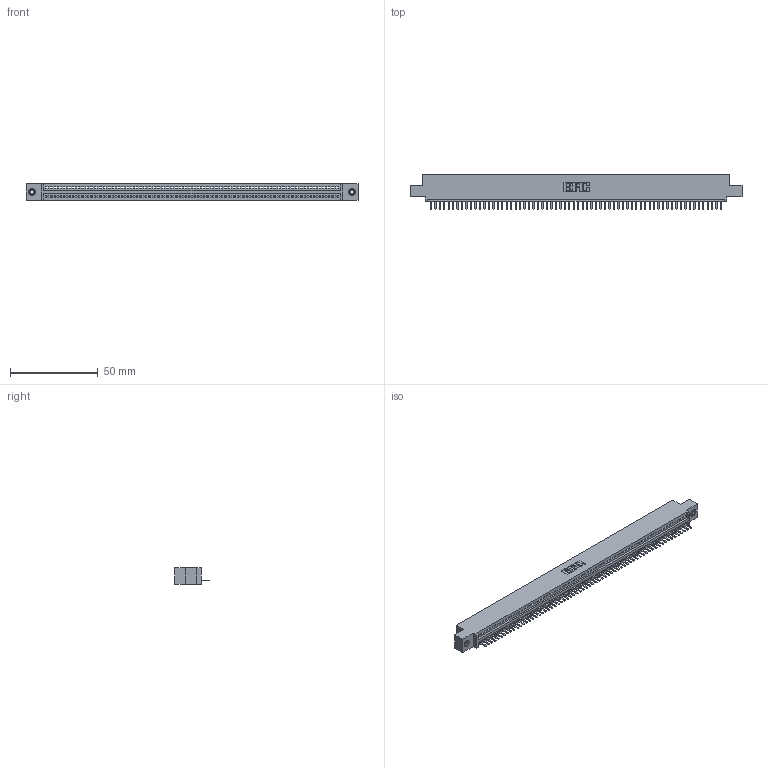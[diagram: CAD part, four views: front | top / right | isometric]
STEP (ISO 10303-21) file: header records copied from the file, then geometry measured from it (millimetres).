
FILE_DESCRIPTION (( 'STEP AP203' ), '1' );
FILE_NAME ('395-066-520-408.STEP', '2018-11-25T00:41:00', ( '' ), ( '' ), 'SwSTEP 2.0', 'SolidWorks 2016', '' );
FILE_SCHEMA (( 'CONFIG_CONTROL_DESIGN' ));
Length unit declared in the file: inch
Products named in the file (4): 345-292-001_345-293-120; 345-250-001_345-250-003-102; 345 Part_0.110 Offset - 0.156 Dia-TI; 395-066-520-408
Assembly tree (69 placements, depth 2):
  395-066-520-408
    345 Part_0.110 Offset - 0.156 Dia-TI
    345-292-001_345-293-120  x66
    345-250-001_345-250-003-102  x2
Bounding box: 188.85 x 19.68 x 9.4 mm (x, y, z)
Volume: 17863.9 mm3; surface area: 23545.7 mm2
Topology: 69 solids, 69 shells, 4282 faces, 12633 edges, 8238 vertices
Faces by surface type: plane 2888, cylinder 1378, cone 12, torus 4
Entity records: 47874 total; most frequent: CARTESIAN_POINT 8285, ORIENTED_EDGE 8266, DIRECTION 7215, EDGE_CURVE 4133, VECTOR 3713, LINE 3713, VERTEX_POINT 2748, AXIS2_PLACEMENT_3D 1751
